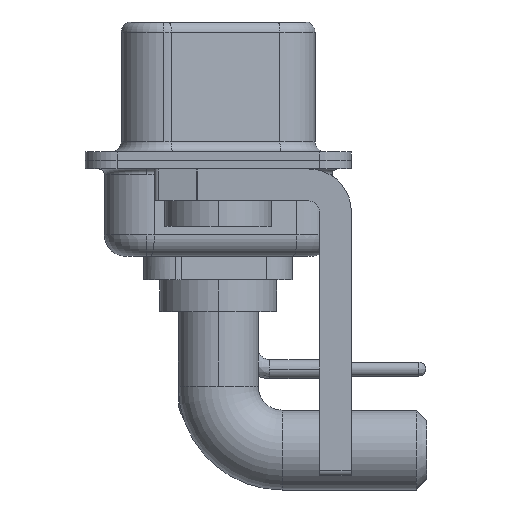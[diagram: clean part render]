
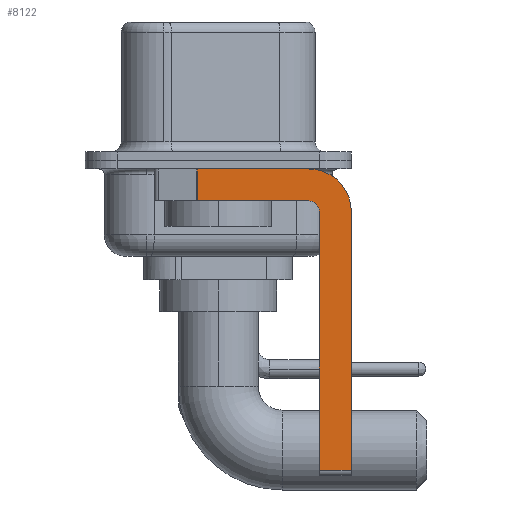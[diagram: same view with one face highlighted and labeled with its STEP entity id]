
A CAD part, left-side view. The second image highlights one B-rep face of the part: STEP entity #8122.
In plain terms, the highlighted planar face has unit normal (-1, 0, 0).
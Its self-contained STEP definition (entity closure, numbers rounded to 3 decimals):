
#92 = DIRECTION ( 'NONE',  ( 0., 0., -1. ) ) ;
#554 = DIRECTION ( 'NONE',  ( 0., 0., -1. ) ) ;
#785 = VERTEX_POINT ( 'NONE', #4882 ) ;
#1132 = DIRECTION ( 'NONE',  ( 1., 0., 0. ) ) ;
#1846 = EDGE_CURVE ( 'NONE', #18385, #11474, #11301, .T. ) ;
#2039 = ORIENTED_EDGE ( 'NONE', *, *, #14339, .F. ) ;
#2174 = CARTESIAN_POINT ( 'NONE',  ( -2.9, -4.75, -14.8 ) ) ;
#2404 = EDGE_LOOP ( 'NONE', ( #18110, #14137, #11466, #2039, #24960, #9590, #5195, #9405 ) ) ;
#2927 = EDGE_CURVE ( 'NONE', #785, #9347, #8454, .T. ) ;
#3224 = VECTOR ( 'NONE', #12099, 1000. ) ;
#3242 = CARTESIAN_POINT ( 'NONE',  ( -2.9, -4.25, -0.4 ) ) ;
#3284 = EDGE_CURVE ( 'NONE', #8681, #11474, #16216, .T. ) ;
#3457 = VERTEX_POINT ( 'NONE', #3242 ) ;
#4180 = CARTESIAN_POINT ( 'NONE',  ( -2.9, -4.25, -14.55 ) ) ;
#4758 = FACE_OUTER_BOUND ( 'NONE', #2404, .T. ) ;
#4767 = CIRCLE ( 'NONE', #8474, 0.5 ) ;
#4882 = CARTESIAN_POINT ( 'NONE',  ( -2.9, -4.75, -14.55 ) ) ;
#5195 = ORIENTED_EDGE ( 'NONE', *, *, #16678, .F. ) ;
#6044 = DIRECTION ( 'NONE',  ( 0., -1., 0. ) ) ;
#6429 = PLANE ( 'NONE',  #17814 ) ;
#7276 = VECTOR ( 'NONE', #554, 1000. ) ;
#8122 = ADVANCED_FACE ( 'NONE', ( #4758 ), #6429, .F. ) ;
#8367 = CARTESIAN_POINT ( 'NONE',  ( -2.9, 3., -0.4 ) ) ;
#8454 = LINE ( 'NONE', #4180, #3224 ) ;
#8474 = AXIS2_PLACEMENT_3D ( 'NONE', #9429, #17221, #15391 ) ;
#8546 = CARTESIAN_POINT ( 'NONE',  ( -2.9, 0.978, -1.9 ) ) ;
#8681 = VERTEX_POINT ( 'NONE', #13018 ) ;
#8846 = CARTESIAN_POINT ( 'NONE',  ( -2.9, 0.978, -1.9 ) ) ;
#9347 = VERTEX_POINT ( 'NONE', #25615 ) ;
#9405 = ORIENTED_EDGE ( 'NONE', *, *, #19373, .F. ) ;
#9429 = CARTESIAN_POINT ( 'NONE',  ( -2.9, -4.25, -2.4 ) ) ;
#9590 = ORIENTED_EDGE ( 'NONE', *, *, #2927, .T. ) ;
#10532 = VERTEX_POINT ( 'NONE', #13505 ) ;
#11301 = LINE ( 'NONE', #21908, #19346 ) ;
#11466 = ORIENTED_EDGE ( 'NONE', *, *, #1846, .F. ) ;
#11474 = VERTEX_POINT ( 'NONE', #8846 ) ;
#12099 = DIRECTION ( 'NONE',  ( 0., -1., 0. ) ) ;
#13018 = CARTESIAN_POINT ( 'NONE',  ( -2.9, 0.978, -0.4 ) ) ;
#13505 = CARTESIAN_POINT ( 'NONE',  ( -2.9, -6.25, -2.4 ) ) ;
#14137 = ORIENTED_EDGE ( 'NONE', *, *, #3284, .T. ) ;
#14301 = VECTOR ( 'NONE', #6044, 1000. ) ;
#14339 = EDGE_CURVE ( 'NONE', #25659, #18385, #4767, .T. ) ;
#14467 = CARTESIAN_POINT ( 'NONE',  ( -2.9, -4.25, -2.4 ) ) ;
#15391 = DIRECTION ( 'NONE',  ( 0., 0., 1. ) ) ;
#15437 = EDGE_CURVE ( 'NONE', #8681, #3457, #21899, .T. ) ;
#15472 = EDGE_CURVE ( 'NONE', #785, #25659, #19700, .T. ) ;
#15776 = DIRECTION ( 'NONE',  ( 1., 0., 0. ) ) ;
#16162 = DIRECTION ( 'NONE',  ( 0., 0., 1. ) ) ;
#16216 = LINE ( 'NONE', #8546, #22398 ) ;
#16483 = DIRECTION ( 'NONE',  ( 0., 0., -1. ) ) ;
#16678 = EDGE_CURVE ( 'NONE', #10532, #9347, #20404, .T. ) ;
#17221 = DIRECTION ( 'NONE',  ( -1., 0., 0. ) ) ;
#17814 = AXIS2_PLACEMENT_3D ( 'NONE', #14467, #1132, #24379 ) ;
#17854 = CARTESIAN_POINT ( 'NONE',  ( -2.9, -4.25, -2.4 ) ) ;
#17915 = CARTESIAN_POINT ( 'NONE',  ( -2.9, -4.25, -1.9 ) ) ;
#18110 = ORIENTED_EDGE ( 'NONE', *, *, #15437, .F. ) ;
#18385 = VERTEX_POINT ( 'NONE', #17915 ) ;
#18825 = CARTESIAN_POINT ( 'NONE',  ( -2.9, -6.25, -2.4 ) ) ;
#19346 = VECTOR ( 'NONE', #25224, 1000. ) ;
#19373 = EDGE_CURVE ( 'NONE', #3457, #10532, #19417, .T. ) ;
#19417 = CIRCLE ( 'NONE', #23971, 2. ) ;
#19700 = LINE ( 'NONE', #2174, #19730 ) ;
#19730 = VECTOR ( 'NONE', #16162, 1000. ) ;
#20404 = LINE ( 'NONE', #18825, #7276 ) ;
#21899 = LINE ( 'NONE', #8367, #14301 ) ;
#21908 = CARTESIAN_POINT ( 'NONE',  ( -2.9, -4.25, -1.9 ) ) ;
#22398 = VECTOR ( 'NONE', #16483, 1000. ) ;
#22798 = CARTESIAN_POINT ( 'NONE',  ( -2.9, -4.75, -2.4 ) ) ;
#23971 = AXIS2_PLACEMENT_3D ( 'NONE', #17854, #15776, #92 ) ;
#24379 = DIRECTION ( 'NONE',  ( 0., 0., -1. ) ) ;
#24960 = ORIENTED_EDGE ( 'NONE', *, *, #15472, .F. ) ;
#25224 = DIRECTION ( 'NONE',  ( 0., 1., 0. ) ) ;
#25615 = CARTESIAN_POINT ( 'NONE',  ( -2.9, -6.25, -14.55 ) ) ;
#25659 = VERTEX_POINT ( 'NONE', #22798 ) ;
